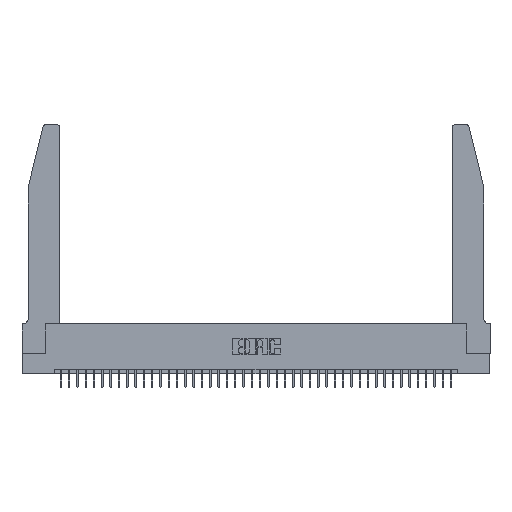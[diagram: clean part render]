
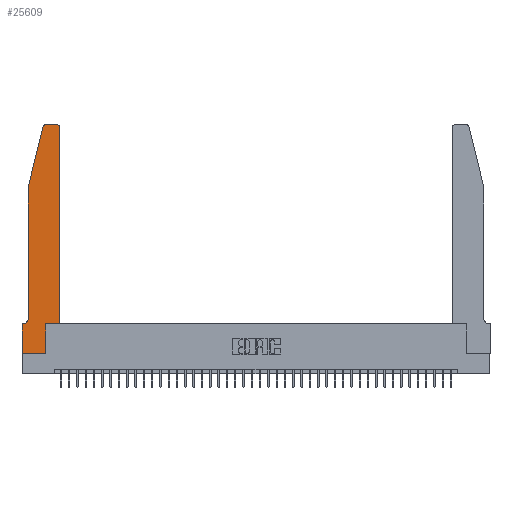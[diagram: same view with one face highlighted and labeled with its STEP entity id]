
A CAD part, top view. The second image highlights one B-rep face of the part: STEP entity #25609.
In plain terms, the highlighted planar face has unit normal (0, 0, 1).
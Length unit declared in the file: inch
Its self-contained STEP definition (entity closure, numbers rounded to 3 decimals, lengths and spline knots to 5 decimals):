
#1203 = EDGE_CURVE ( 'NONE', #14404, #19226, #21168, .T. ) ;
#1651 = AXIS2_PLACEMENT_3D ( 'NONE', #18237, #40639, #21513 ) ;
#1797 = VECTOR ( 'NONE', #27493, 39.37008 ) ;
#2244 = ORIENTED_EDGE ( 'NONE', *, *, #31291, .T. ) ;
#2640 = CARTESIAN_POINT ( 'NONE',  ( 0.0055, 0.42, 0.37 ) ) ;
#2761 = VERTEX_POINT ( 'NONE', #38625 ) ;
#3144 = AXIS2_PLACEMENT_3D ( 'NONE', #37400, #18219, #40621 ) ;
#4150 = EDGE_CURVE ( 'NONE', #35026, #6158, #27407, .T. ) ;
#4267 = VERTEX_POINT ( 'NONE', #7545 ) ;
#4586 = LINE ( 'NONE', #37552, #37854 ) ;
#5102 = EDGE_CURVE ( 'NONE', #35020, #8617, #19340, .T. ) ;
#5685 = VECTOR ( 'NONE', #38711, 39.37008 ) ;
#5848 = ORIENTED_EDGE ( 'NONE', *, *, #15563, .T. ) ;
#5864 = DIRECTION ( 'NONE',  ( -1., 0., 0. ) ) ;
#6158 = VERTEX_POINT ( 'NONE', #24286 ) ;
#6473 = AXIS2_PLACEMENT_3D ( 'NONE', #18008, #14857, #37329 ) ;
#6506 = CARTESIAN_POINT ( 'NONE',  ( 0.4505, 2.72, 0.37 ) ) ;
#6761 = ORIENTED_EDGE ( 'NONE', *, *, #21453, .T. ) ;
#7031 = CARTESIAN_POINT ( 'NONE',  ( 0.0755, 2., 0.37 ) ) ;
#7168 = CARTESIAN_POINT ( 'NONE',  ( 0.2865, 0., 0.37 ) ) ;
#7170 = VECTOR ( 'NONE', #32234, 39.37008 ) ;
#7545 = CARTESIAN_POINT ( 'NONE',  ( 0.25487, 2.72718, 0.37 ) ) ;
#8240 = ORIENTED_EDGE ( 'NONE', *, *, #4150, .T. ) ;
#8284 = ORIENTED_EDGE ( 'NONE', *, *, #30619, .T. ) ;
#8318 = PLANE ( 'NONE',  #6473 ) ;
#8617 = VERTEX_POINT ( 'NONE', #15407 ) ;
#8947 = VECTOR ( 'NONE', #28533, 39.37008 ) ;
#10242 = DIRECTION ( 'NONE',  ( 0., -1., 0. ) ) ;
#10308 = EDGE_CURVE ( 'NONE', #19226, #12490, #22063, .T. ) ;
#10414 = LINE ( 'NONE', #21047, #1797 ) ;
#10660 = VECTOR ( 'NONE', #24362, 39.37008 ) ;
#11054 = ORIENTED_EDGE ( 'NONE', *, *, #1203, .T. ) ;
#11065 = CARTESIAN_POINT ( 'NONE',  ( 0., 0.35, 0.37 ) ) ;
#12490 = VERTEX_POINT ( 'NONE', #34392 ) ;
#12924 = ORIENTED_EDGE ( 'NONE', *, *, #27132, .T. ) ;
#12930 = CARTESIAN_POINT ( 'NONE',  ( 0.4505, 0.35, 0.37 ) ) ;
#14404 = VERTEX_POINT ( 'NONE', #28710 ) ;
#14788 = LINE ( 'NONE', #12930, #7170 ) ;
#14857 = DIRECTION ( 'NONE',  ( 0., 0., 1. ) ) ;
#15407 = CARTESIAN_POINT ( 'NONE',  ( 0.2865, 0.35, 0.37 ) ) ;
#15563 = EDGE_CURVE ( 'NONE', #40841, #2761, #23891, .T. ) ;
#15587 = EDGE_CURVE ( 'NONE', #34841, #40841, #4586, .T. ) ;
#17422 = CARTESIAN_POINT ( 'NONE',  ( 0., 0., 0.37 ) ) ;
#18008 = CARTESIAN_POINT ( 'NONE',  ( 0., 0.35, 0.37 ) ) ;
#18219 = DIRECTION ( 'NONE',  ( 0., 0., 1. ) ) ;
#18237 = CARTESIAN_POINT ( 'NONE',  ( 0.4205, 2.72, 0.37 ) ) ;
#18686 = CIRCLE ( 'NONE', #31404, 0.07 ) ;
#18845 = VECTOR ( 'NONE', #10242, 39.37008 ) ;
#19226 = VERTEX_POINT ( 'NONE', #11065 ) ;
#19340 = LINE ( 'NONE', #37052, #10660 ) ;
#20148 = EDGE_CURVE ( 'NONE', #4267, #35026, #35665, .T. ) ;
#21047 = CARTESIAN_POINT ( 'NONE',  ( 0.2605, 2.75, 0.37 ) ) ;
#21168 = LINE ( 'NONE', #27238, #37141 ) ;
#21323 = EDGE_LOOP ( 'NONE', ( #39045, #6761, #38332, #8240, #12924, #11054, #37290, #8284, #34110, #2244, #27918, #5848 ) ) ;
#21453 = EDGE_CURVE ( 'NONE', #32127, #4267, #30566, .T. ) ;
#21513 = DIRECTION ( 'NONE',  ( 1., 0., 0. ) ) ;
#21997 = LINE ( 'NONE', #29095, #5685 ) ;
#22063 = LINE ( 'NONE', #17422, #28580 ) ;
#23166 = CARTESIAN_POINT ( 'NONE',  ( 0.0755, 2., 0.37 ) ) ;
#23891 = CIRCLE ( 'NONE', #1651, 0.03 ) ;
#24286 = CARTESIAN_POINT ( 'NONE',  ( 0.0755, 0.42, 0.37 ) ) ;
#24362 = DIRECTION ( 'NONE',  ( 0., 1., 0. ) ) ;
#25328 = CARTESIAN_POINT ( 'NONE',  ( 0.0755, 2., 0.37 ) ) ;
#25337 = DIRECTION ( 'NONE',  ( 0., 0., -1. ) ) ;
#25609 = ADVANCED_FACE ( 'NONE', ( #32349 ), #8318, .T. ) ;
#27132 = EDGE_CURVE ( 'NONE', #6158, #14404, #18686, .T. ) ;
#27137 = DIRECTION ( 'NONE',  ( 0., -1., 0. ) ) ;
#27238 = CARTESIAN_POINT ( 'NONE',  ( 0.0755, 0.35, 0.37 ) ) ;
#27407 = LINE ( 'NONE', #23166, #18845 ) ;
#27493 = DIRECTION ( 'NONE',  ( -1., 0., 0. ) ) ;
#27918 = ORIENTED_EDGE ( 'NONE', *, *, #15587, .T. ) ;
#28094 = DIRECTION ( 'NONE',  ( 0., 1., 0. ) ) ;
#28179 = EDGE_CURVE ( 'NONE', #2761, #32127, #10414, .T. ) ;
#28533 = DIRECTION ( 'NONE',  ( -0.239, -0.971, 0. ) ) ;
#28580 = VECTOR ( 'NONE', #27137, 39.37008 ) ;
#28710 = CARTESIAN_POINT ( 'NONE',  ( 0.0055, 0.35, 0.37 ) ) ;
#29095 = CARTESIAN_POINT ( 'NONE',  ( 0., 0., 0.37 ) ) ;
#30566 = CIRCLE ( 'NONE', #3144, 0.03 ) ;
#30619 = EDGE_CURVE ( 'NONE', #12490, #35020, #21997, .T. ) ;
#31291 = EDGE_CURVE ( 'NONE', #8617, #34841, #14788, .T. ) ;
#31404 = AXIS2_PLACEMENT_3D ( 'NONE', #2640, #25337, #5864 ) ;
#32127 = VERTEX_POINT ( 'NONE', #33289 ) ;
#32234 = DIRECTION ( 'NONE',  ( 1., 0., 0. ) ) ;
#32349 = FACE_OUTER_BOUND ( 'NONE', #21323, .T. ) ;
#33289 = CARTESIAN_POINT ( 'NONE',  ( 0.284, 2.75, 0.37 ) ) ;
#33648 = DIRECTION ( 'NONE',  ( -1., 0., 0. ) ) ;
#34110 = ORIENTED_EDGE ( 'NONE', *, *, #5102, .T. ) ;
#34392 = CARTESIAN_POINT ( 'NONE',  ( 0., 0., 0.37 ) ) ;
#34841 = VERTEX_POINT ( 'NONE', #35226 ) ;
#35020 = VERTEX_POINT ( 'NONE', #7168 ) ;
#35026 = VERTEX_POINT ( 'NONE', #7031 ) ;
#35226 = CARTESIAN_POINT ( 'NONE',  ( 0.4505, 0.35, 0.37 ) ) ;
#35665 = LINE ( 'NONE', #25328, #8947 ) ;
#37052 = CARTESIAN_POINT ( 'NONE',  ( 0.2865, 0.35, 0.37 ) ) ;
#37141 = VECTOR ( 'NONE', #33648, 39.37008 ) ;
#37290 = ORIENTED_EDGE ( 'NONE', *, *, #10308, .T. ) ;
#37329 = DIRECTION ( 'NONE',  ( 1., 0., 0. ) ) ;
#37400 = CARTESIAN_POINT ( 'NONE',  ( 0.284, 2.72, 0.37 ) ) ;
#37552 = CARTESIAN_POINT ( 'NONE',  ( 0.4505, 0.35, 0.37 ) ) ;
#37854 = VECTOR ( 'NONE', #28094, 39.37008 ) ;
#38332 = ORIENTED_EDGE ( 'NONE', *, *, #20148, .T. ) ;
#38625 = CARTESIAN_POINT ( 'NONE',  ( 0.4205, 2.75, 0.37 ) ) ;
#38711 = DIRECTION ( 'NONE',  ( 1., 0., 0. ) ) ;
#39045 = ORIENTED_EDGE ( 'NONE', *, *, #28179, .T. ) ;
#40621 = DIRECTION ( 'NONE',  ( 1., 0., 0. ) ) ;
#40639 = DIRECTION ( 'NONE',  ( 0., 0., 1. ) ) ;
#40841 = VERTEX_POINT ( 'NONE', #6506 ) ;
